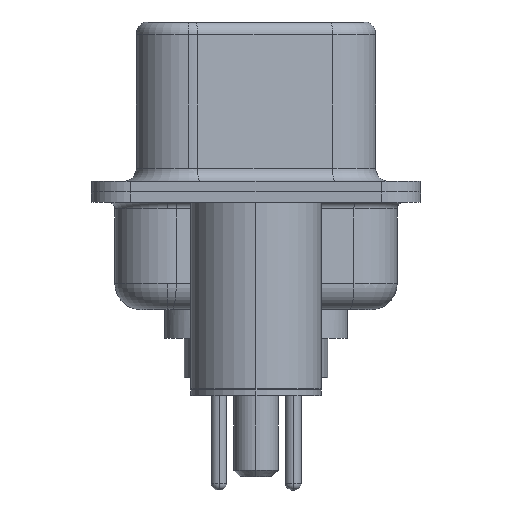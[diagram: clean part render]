
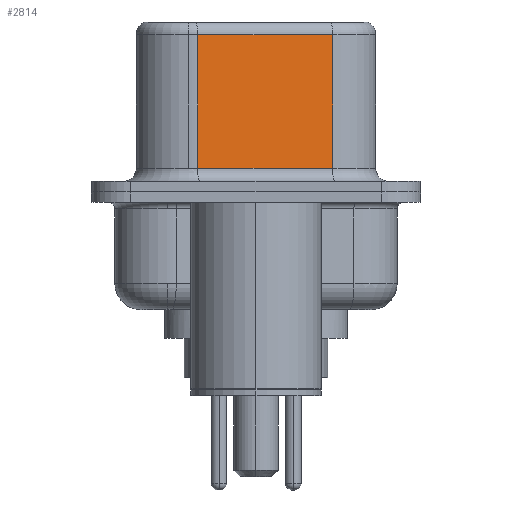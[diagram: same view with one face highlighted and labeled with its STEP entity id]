
A CAD part, left-side view. The second image highlights one B-rep face of the part: STEP entity #2814.
In plain terms, the highlighted planar face has unit normal (-0.985, -0.174, 0).
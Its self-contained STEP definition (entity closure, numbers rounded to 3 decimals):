
#345 = VERTEX_POINT ( 'NONE', #12338 ) ;
#592 = CARTESIAN_POINT ( 'NONE',  ( 4.565, -2.927, 0.9 ) ) ;
#1806 = LINE ( 'NONE', #592, #14602 ) ;
#1809 = LINE ( 'NONE', #12454, #18904 ) ;
#2050 = LINE ( 'NONE', #17311, #19161 ) ;
#2814 = ADVANCED_FACE ( 'NONE', ( #20189 ), #10595, .F. ) ;
#3444 = VECTOR ( 'NONE', #20441, 1000. ) ;
#4089 = DIRECTION ( 'NONE',  ( 0., 0., -1. ) ) ;
#4642 = VERTEX_POINT ( 'NONE', #12482 ) ;
#5309 = ORIENTED_EDGE ( 'NONE', *, *, #17208, .T. ) ;
#6845 = EDGE_CURVE ( 'NONE', #345, #4642, #16228, .T. ) ;
#7304 = DIRECTION ( 'NONE',  ( 0.174, -0.985, 0. ) ) ;
#7922 = VERTEX_POINT ( 'NONE', #8319 ) ;
#8302 = EDGE_CURVE ( 'NONE', #345, #7922, #2050, .T. ) ;
#8319 = CARTESIAN_POINT ( 'NONE',  ( 4.565, -2.927, 0.9 ) ) ;
#8603 = CARTESIAN_POINT ( 'NONE',  ( 3.655, 2.233, 0.9 ) ) ;
#8842 = ORIENTED_EDGE ( 'NONE', *, *, #6845, .T. ) ;
#9029 = ORIENTED_EDGE ( 'NONE', *, *, #9599, .T. ) ;
#9599 = EDGE_CURVE ( 'NONE', #10552, #7922, #1806, .T. ) ;
#10552 = VERTEX_POINT ( 'NONE', #8603 ) ;
#10595 = PLANE ( 'NONE',  #17551 ) ;
#11384 = CARTESIAN_POINT ( 'NONE',  ( 4.565, -2.927, 6.52 ) ) ;
#12338 = CARTESIAN_POINT ( 'NONE',  ( 4.565, -2.927, 6.02 ) ) ;
#12454 = CARTESIAN_POINT ( 'NONE',  ( 3.655, 2.233, 6.52 ) ) ;
#12482 = CARTESIAN_POINT ( 'NONE',  ( 3.655, 2.233, 6.02 ) ) ;
#12584 = EDGE_LOOP ( 'NONE', ( #15728, #8842, #5309, #9029 ) ) ;
#12615 = DIRECTION ( 'NONE',  ( 0.985, 0.174, 0. ) ) ;
#13716 = DIRECTION ( 'NONE',  ( -0.174, 0.985, 0. ) ) ;
#14051 = DIRECTION ( 'NONE',  ( 0., 0., -1. ) ) ;
#14602 = VECTOR ( 'NONE', #7304, 1000. ) ;
#15728 = ORIENTED_EDGE ( 'NONE', *, *, #8302, .F. ) ;
#16228 = LINE ( 'NONE', #18994, #3444 ) ;
#17208 = EDGE_CURVE ( 'NONE', #4642, #10552, #1809, .T. ) ;
#17311 = CARTESIAN_POINT ( 'NONE',  ( 4.565, -2.927, 6.52 ) ) ;
#17551 = AXIS2_PLACEMENT_3D ( 'NONE', #11384, #12615, #13716 ) ;
#18904 = VECTOR ( 'NONE', #14051, 1000. ) ;
#18994 = CARTESIAN_POINT ( 'NONE',  ( 4.565, -2.927, 6.02 ) ) ;
#19161 = VECTOR ( 'NONE', #4089, 1000. ) ;
#20189 = FACE_OUTER_BOUND ( 'NONE', #12584, .T. ) ;
#20441 = DIRECTION ( 'NONE',  ( -0.174, 0.985, 0. ) ) ;
